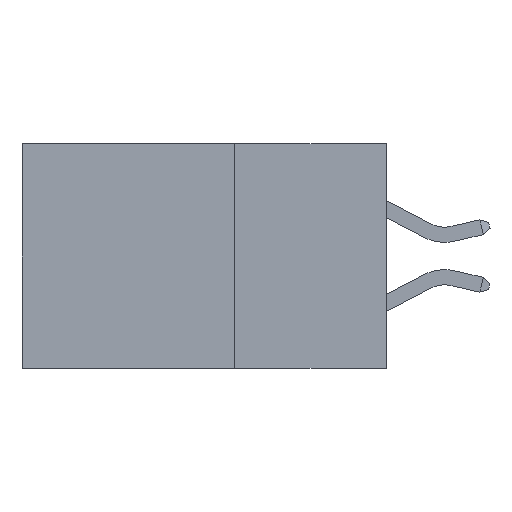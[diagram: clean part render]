
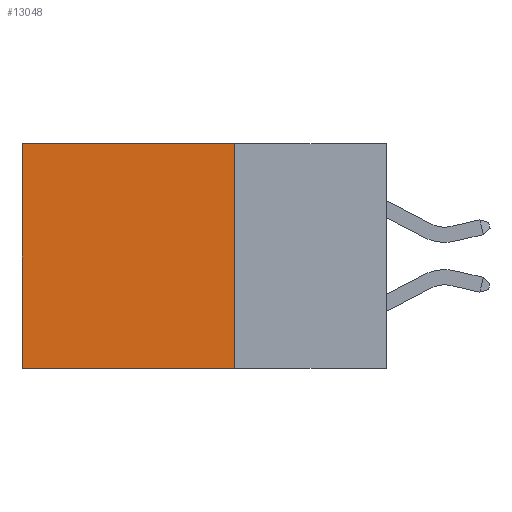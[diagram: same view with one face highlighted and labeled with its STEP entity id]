
A CAD part, left-side view. The second image highlights one B-rep face of the part: STEP entity #13048.
In plain terms, the highlighted planar face has unit normal (-1, 0, 0).
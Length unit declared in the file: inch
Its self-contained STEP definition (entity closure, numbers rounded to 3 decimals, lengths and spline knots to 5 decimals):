
#225 = VECTOR ( 'NONE', #4630, 39.37008 ) ;
#976 = LINE ( 'NONE', #11250, #12813 ) ;
#1627 = CARTESIAN_POINT ( 'NONE',  ( 0.2615, 0.25, 0. ) ) ;
#2071 = CARTESIAN_POINT ( 'NONE',  ( 0.2615, 0.25, -0.37 ) ) ;
#2707 = VERTEX_POINT ( 'NONE', #12510 ) ;
#3204 = EDGE_CURVE ( 'NONE', #17602, #8151, #8636, .T. ) ;
#4630 = DIRECTION ( 'NONE',  ( 0., 1., 0. ) ) ;
#4807 = AXIS2_PLACEMENT_3D ( 'NONE', #15361, #17169, #20878 ) ;
#6656 = EDGE_CURVE ( 'NONE', #8151, #2707, #976, .T. ) ;
#7726 = CARTESIAN_POINT ( 'NONE',  ( 0.2615, 0.25, -0.37 ) ) ;
#8151 = VERTEX_POINT ( 'NONE', #19032 ) ;
#8544 = DIRECTION ( 'NONE',  ( 0., 0., -1. ) ) ;
#8636 = LINE ( 'NONE', #1627, #8759 ) ;
#8697 = FACE_OUTER_BOUND ( 'NONE', #15075, .T. ) ;
#8759 = VECTOR ( 'NONE', #15637, 39.37008 ) ;
#9387 = ORIENTED_EDGE ( 'NONE', *, *, #3204, .T. ) ;
#10160 = PLANE ( 'NONE',  #4807 ) ;
#10743 = EDGE_CURVE ( 'NONE', #17602, #20525, #20485, .T. ) ;
#11250 = CARTESIAN_POINT ( 'NONE',  ( 0.2615, 0.6, -0.37 ) ) ;
#11899 = ORIENTED_EDGE ( 'NONE', *, *, #6656, .T. ) ;
#12255 = CARTESIAN_POINT ( 'NONE',  ( 0.2615, 0.25, -0.37 ) ) ;
#12510 = CARTESIAN_POINT ( 'NONE',  ( 0.2615, 0.6, -0.37 ) ) ;
#12813 = VECTOR ( 'NONE', #21292, 39.37008 ) ;
#13048 = ADVANCED_FACE ( 'NONE', ( #8697 ), #10160, .F. ) ;
#15075 = EDGE_LOOP ( 'NONE', ( #11899, #20843, #16732, #9387 ) ) ;
#15361 = CARTESIAN_POINT ( 'NONE',  ( 0.2615, 0.25, -0.37 ) ) ;
#15637 = DIRECTION ( 'NONE',  ( 0., 1., 0. ) ) ;
#16700 = VECTOR ( 'NONE', #8544, 39.37008 ) ;
#16732 = ORIENTED_EDGE ( 'NONE', *, *, #10743, .F. ) ;
#17169 = DIRECTION ( 'NONE',  ( 1., 0., 0. ) ) ;
#17213 = CARTESIAN_POINT ( 'NONE',  ( 0.2615, 0.25, 0. ) ) ;
#17602 = VERTEX_POINT ( 'NONE', #17213 ) ;
#19032 = CARTESIAN_POINT ( 'NONE',  ( 0.2615, 0.6, 0. ) ) ;
#19889 = LINE ( 'NONE', #7726, #225 ) ;
#20485 = LINE ( 'NONE', #2071, #16700 ) ;
#20525 = VERTEX_POINT ( 'NONE', #12255 ) ;
#20843 = ORIENTED_EDGE ( 'NONE', *, *, #22286, .F. ) ;
#20878 = DIRECTION ( 'NONE',  ( 0., 0., -1. ) ) ;
#21292 = DIRECTION ( 'NONE',  ( 0., 0., -1. ) ) ;
#22286 = EDGE_CURVE ( 'NONE', #20525, #2707, #19889, .T. ) ;
